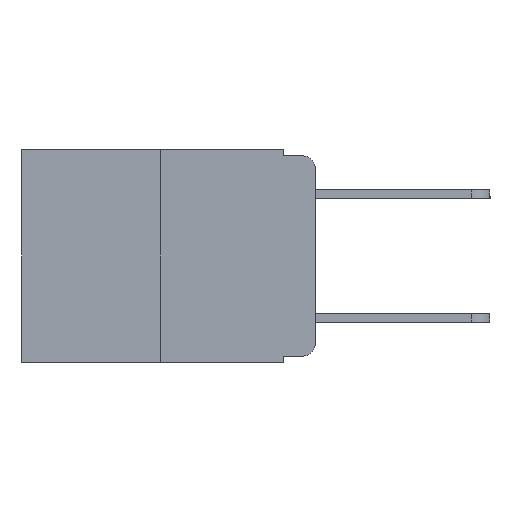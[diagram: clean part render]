
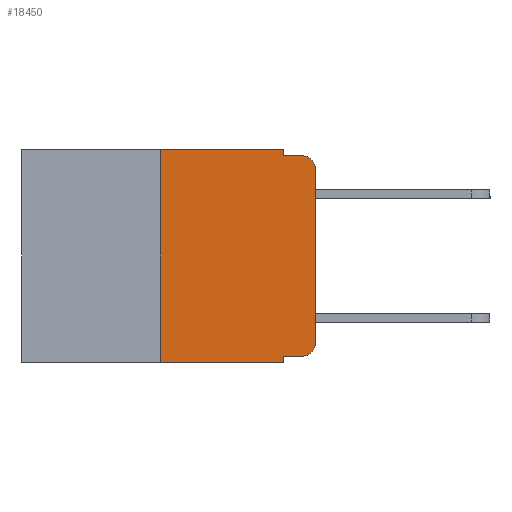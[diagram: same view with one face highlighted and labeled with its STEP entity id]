
A CAD part, left-side view. The second image highlights one B-rep face of the part: STEP entity #18450.
In plain terms, the highlighted planar face has unit normal (-1, 0, 0).
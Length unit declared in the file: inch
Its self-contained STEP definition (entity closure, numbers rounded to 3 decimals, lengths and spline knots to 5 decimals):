
#260 = CARTESIAN_POINT ( 'NONE',  ( 0., 0.051, -0.333 ) ) ;
#390 = CARTESIAN_POINT ( 'NONE',  ( 0., 0.051, 0. ) ) ;
#665 = VERTEX_POINT ( 'NONE', #9069 ) ;
#794 = CARTESIAN_POINT ( 'NONE',  ( 0., 0.25, 0. ) ) ;
#866 = VERTEX_POINT ( 'NONE', #12748 ) ;
#875 = VECTOR ( 'NONE', #21297, 39.37008 ) ;
#1128 = EDGE_CURVE ( 'NONE', #5649, #866, #7113, .T. ) ;
#1184 = ORIENTED_EDGE ( 'NONE', *, *, #2465, .T. ) ;
#1261 = ORIENTED_EDGE ( 'NONE', *, *, #1128, .T. ) ;
#1304 = CARTESIAN_POINT ( 'NONE',  ( 0., 0.473, -0.343 ) ) ;
#1504 = LINE ( 'NONE', #2951, #875 ) ;
#1678 = ORIENTED_EDGE ( 'NONE', *, *, #21907, .F. ) ;
#1726 = ORIENTED_EDGE ( 'NONE', *, *, #17833, .F. ) ;
#2394 = VECTOR ( 'NONE', #6942, 39.37008 ) ;
#2465 = EDGE_CURVE ( 'NONE', #665, #5649, #20380, .T. ) ;
#2655 = EDGE_CURVE ( 'NONE', #5919, #11666, #2701, .T. ) ;
#2701 = LINE ( 'NONE', #15028, #19641 ) ;
#2951 = CARTESIAN_POINT ( 'NONE',  ( 0., 0.051, 0. ) ) ;
#3430 = CIRCLE ( 'NONE', #18478, 0.02 ) ;
#3949 = CARTESIAN_POINT ( 'NONE',  ( 0., 0.051, 0. ) ) ;
#4670 = LINE ( 'NONE', #3949, #8776 ) ;
#4866 = LINE ( 'NONE', #19600, #20856 ) ;
#5419 = VERTEX_POINT ( 'NONE', #12773 ) ;
#5501 = DIRECTION ( 'NONE',  ( -1., 0., 0. ) ) ;
#5580 = VECTOR ( 'NONE', #13751, 39.37008 ) ;
#5649 = VERTEX_POINT ( 'NONE', #18687 ) ;
#5919 = VERTEX_POINT ( 'NONE', #6114 ) ;
#6114 = CARTESIAN_POINT ( 'NONE',  ( 0., 0.25, 0. ) ) ;
#6342 = VECTOR ( 'NONE', #6607, 39.37008 ) ;
#6405 = AXIS2_PLACEMENT_3D ( 'NONE', #11988, #5501, #7182 ) ;
#6607 = DIRECTION ( 'NONE',  ( 0., 0., 1. ) ) ;
#6665 = ORIENTED_EDGE ( 'NONE', *, *, #2655, .F. ) ;
#6942 = DIRECTION ( 'NONE',  ( 0., 0., 1. ) ) ;
#7113 = CIRCLE ( 'NONE', #6405, 0.02 ) ;
#7117 = VECTOR ( 'NONE', #15614, 39.37008 ) ;
#7182 = DIRECTION ( 'NONE',  ( 0., 0., -1. ) ) ;
#7226 = CARTESIAN_POINT ( 'NONE',  ( 0., 0., 0. ) ) ;
#7721 = EDGE_CURVE ( 'NONE', #5419, #11145, #14594, .T. ) ;
#8414 = VERTEX_POINT ( 'NONE', #11660 ) ;
#8776 = VECTOR ( 'NONE', #14258, 39.37008 ) ;
#8782 = DIRECTION ( 'NONE',  ( 1., 0., 0. ) ) ;
#9069 = CARTESIAN_POINT ( 'NONE',  ( 0., 0., -0.313 ) ) ;
#9604 = ORIENTED_EDGE ( 'NONE', *, *, #16790, .F. ) ;
#9693 = VERTEX_POINT ( 'NONE', #260 ) ;
#9710 = CARTESIAN_POINT ( 'NONE',  ( 0., 0.02, -0.333 ) ) ;
#10097 = EDGE_CURVE ( 'NONE', #20419, #665, #3430, .T. ) ;
#10628 = CARTESIAN_POINT ( 'NONE',  ( 0., 0.02, -0.313 ) ) ;
#11145 = VERTEX_POINT ( 'NONE', #18581 ) ;
#11235 = EDGE_CURVE ( 'NONE', #9693, #20419, #11609, .T. ) ;
#11254 = ORIENTED_EDGE ( 'NONE', *, *, #7721, .T. ) ;
#11307 = ORIENTED_EDGE ( 'NONE', *, *, #15728, .F. ) ;
#11572 = ORIENTED_EDGE ( 'NONE', *, *, #11235, .T. ) ;
#11596 = ORIENTED_EDGE ( 'NONE', *, *, #10097, .T. ) ;
#11609 = LINE ( 'NONE', #20248, #7117 ) ;
#11660 = CARTESIAN_POINT ( 'NONE',  ( 0., 0.051, -0.01 ) ) ;
#11666 = VERTEX_POINT ( 'NONE', #390 ) ;
#11988 = CARTESIAN_POINT ( 'NONE',  ( 0., 0.02, -0.03 ) ) ;
#12357 = DIRECTION ( 'NONE',  ( 0., 0., -1. ) ) ;
#12748 = CARTESIAN_POINT ( 'NONE',  ( 0., 0.02, -0.01 ) ) ;
#12773 = CARTESIAN_POINT ( 'NONE',  ( 0., 0.25, -0.343 ) ) ;
#13751 = DIRECTION ( 'NONE',  ( 0., -1., 0. ) ) ;
#13927 = FACE_OUTER_BOUND ( 'NONE', #15615, .T. ) ;
#14258 = DIRECTION ( 'NONE',  ( 0., 0., -1. ) ) ;
#14594 = LINE ( 'NONE', #1304, #5580 ) ;
#15028 = CARTESIAN_POINT ( 'NONE',  ( 0., 0.473, 0. ) ) ;
#15614 = DIRECTION ( 'NONE',  ( 0., -1., 0. ) ) ;
#15615 = EDGE_LOOP ( 'NONE', ( #1184, #1261, #1678, #1726, #6665, #9604, #11254, #11307, #11572, #11596 ) ) ;
#15728 = EDGE_CURVE ( 'NONE', #9693, #11145, #4670, .T. ) ;
#15812 = LINE ( 'NONE', #794, #6342 ) ;
#16790 = EDGE_CURVE ( 'NONE', #5419, #5919, #15812, .T. ) ;
#17100 = AXIS2_PLACEMENT_3D ( 'NONE', #20104, #8782, #20164 ) ;
#17833 = EDGE_CURVE ( 'NONE', #11666, #8414, #1504, .T. ) ;
#17960 = DIRECTION ( 'NONE',  ( 0., -1., 0. ) ) ;
#18450 = ADVANCED_FACE ( 'NONE', ( #13927 ), #18627, .F. ) ;
#18478 = AXIS2_PLACEMENT_3D ( 'NONE', #10628, #21811, #12357 ) ;
#18581 = CARTESIAN_POINT ( 'NONE',  ( 0., 0.051, -0.343 ) ) ;
#18627 = PLANE ( 'NONE',  #17100 ) ;
#18687 = CARTESIAN_POINT ( 'NONE',  ( 0., 0., -0.03 ) ) ;
#19600 = CARTESIAN_POINT ( 'NONE',  ( 0., 0.051, -0.01 ) ) ;
#19641 = VECTOR ( 'NONE', #17960, 39.37008 ) ;
#20104 = CARTESIAN_POINT ( 'NONE',  ( 0., 0.473, 0. ) ) ;
#20164 = DIRECTION ( 'NONE',  ( 0., 0., -1. ) ) ;
#20248 = CARTESIAN_POINT ( 'NONE',  ( 0., 0.051, -0.333 ) ) ;
#20380 = LINE ( 'NONE', #7226, #2394 ) ;
#20419 = VERTEX_POINT ( 'NONE', #9710 ) ;
#20856 = VECTOR ( 'NONE', #21140, 39.37008 ) ;
#21140 = DIRECTION ( 'NONE',  ( 0., -1., 0. ) ) ;
#21297 = DIRECTION ( 'NONE',  ( 0., 0., -1. ) ) ;
#21811 = DIRECTION ( 'NONE',  ( -1., 0., 0. ) ) ;
#21907 = EDGE_CURVE ( 'NONE', #8414, #866, #4866, .T. ) ;
